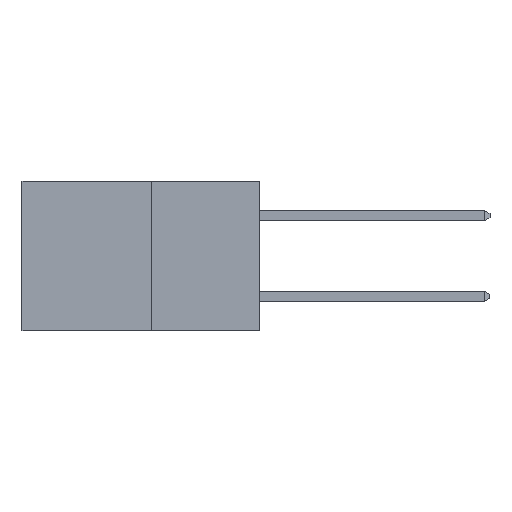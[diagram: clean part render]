
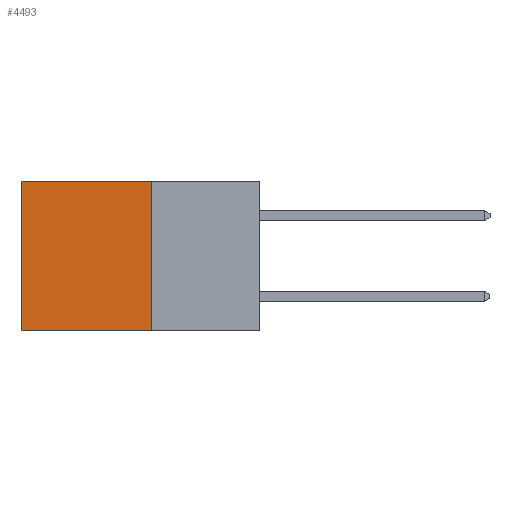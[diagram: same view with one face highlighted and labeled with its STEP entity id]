
A CAD part, left-side view. The second image highlights one B-rep face of the part: STEP entity #4493.
In plain terms, the highlighted planar face has unit normal (-1, 0, 0).
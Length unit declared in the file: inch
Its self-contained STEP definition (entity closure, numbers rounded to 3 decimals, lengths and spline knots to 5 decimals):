
#788 = EDGE_CURVE ( 'NONE', #3824, #1859, #4075, .T. ) ;
#972 = ORIENTED_EDGE ( 'NONE', *, *, #1715, .T. ) ;
#1007 = ORIENTED_EDGE ( 'NONE', *, *, #5031, .F. ) ;
#1356 = DIRECTION ( 'NONE',  ( 1., 0., 0. ) ) ;
#1452 = CARTESIAN_POINT ( 'NONE',  ( 0.277, 0.27, -0.37 ) ) ;
#1570 = AXIS2_PLACEMENT_3D ( 'NONE', #1452, #1356, #3073 ) ;
#1585 = CARTESIAN_POINT ( 'NONE',  ( 0.277, 0.27, -0.37 ) ) ;
#1714 = VECTOR ( 'NONE', #7102, 39.37008 ) ;
#1715 = EDGE_CURVE ( 'NONE', #1859, #5239, #6223, .T. ) ;
#1859 = VERTEX_POINT ( 'NONE', #6448 ) ;
#2606 = FACE_OUTER_BOUND ( 'NONE', #4668, .T. ) ;
#3073 = DIRECTION ( 'NONE',  ( 0., 0., -1. ) ) ;
#3235 = CARTESIAN_POINT ( 'NONE',  ( 0.277, 0.27, 0. ) ) ;
#3597 = ORIENTED_EDGE ( 'NONE', *, *, #4867, .F. ) ;
#3824 = VERTEX_POINT ( 'NONE', #3235 ) ;
#3893 = CARTESIAN_POINT ( 'NONE',  ( 0.277, 0.27, -0.37 ) ) ;
#4075 = LINE ( 'NONE', #7770, #7144 ) ;
#4475 = DIRECTION ( 'NONE',  ( 0., 1., 0. ) ) ;
#4493 = ADVANCED_FACE ( 'NONE', ( #2606 ), #5646, .F. ) ;
#4588 = VECTOR ( 'NONE', #5493, 39.37008 ) ;
#4668 = EDGE_LOOP ( 'NONE', ( #972, #3597, #1007, #5928 ) ) ;
#4867 = EDGE_CURVE ( 'NONE', #6136, #5239, #5248, .T. ) ;
#5026 = CARTESIAN_POINT ( 'NONE',  ( 0.277, 0.59, -0.37 ) ) ;
#5031 = EDGE_CURVE ( 'NONE', #3824, #6136, #6427, .T. ) ;
#5239 = VERTEX_POINT ( 'NONE', #5430 ) ;
#5248 = LINE ( 'NONE', #1585, #6570 ) ;
#5430 = CARTESIAN_POINT ( 'NONE',  ( 0.277, 0.59, -0.37 ) ) ;
#5493 = DIRECTION ( 'NONE',  ( 0., 0., -1. ) ) ;
#5646 = PLANE ( 'NONE',  #1570 ) ;
#5928 = ORIENTED_EDGE ( 'NONE', *, *, #788, .T. ) ;
#6136 = VERTEX_POINT ( 'NONE', #3893 ) ;
#6180 = DIRECTION ( 'NONE',  ( 0., 1., 0. ) ) ;
#6223 = LINE ( 'NONE', #5026, #4588 ) ;
#6427 = LINE ( 'NONE', #7110, #1714 ) ;
#6448 = CARTESIAN_POINT ( 'NONE',  ( 0.277, 0.59, 0. ) ) ;
#6570 = VECTOR ( 'NONE', #4475, 39.37008 ) ;
#7102 = DIRECTION ( 'NONE',  ( 0., 0., -1. ) ) ;
#7110 = CARTESIAN_POINT ( 'NONE',  ( 0.277, 0.27, -0.37 ) ) ;
#7144 = VECTOR ( 'NONE', #6180, 39.37008 ) ;
#7770 = CARTESIAN_POINT ( 'NONE',  ( 0.277, 0.27, 0. ) ) ;
